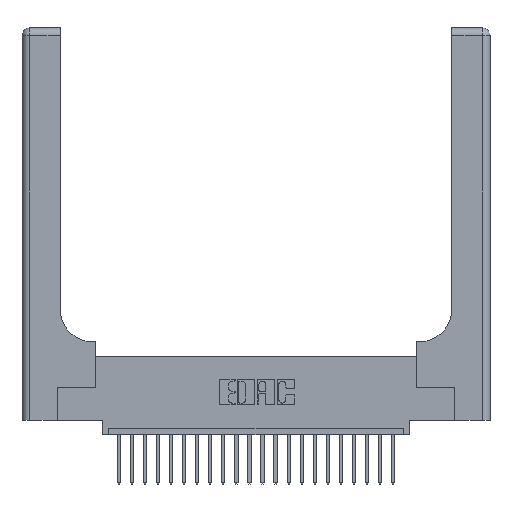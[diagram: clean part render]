
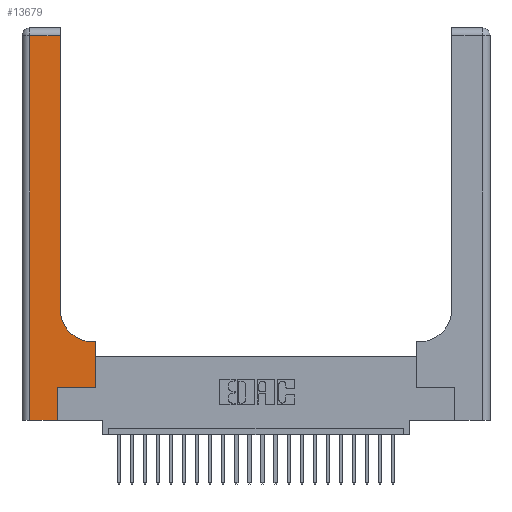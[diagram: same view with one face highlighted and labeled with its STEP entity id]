
A CAD part, top view. The second image highlights one B-rep face of the part: STEP entity #13679.
In plain terms, the highlighted planar face has unit normal (0, 0, 1).
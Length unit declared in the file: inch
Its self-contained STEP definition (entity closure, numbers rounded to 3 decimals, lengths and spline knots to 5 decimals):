
#112 = LINE ( 'NONE', #12360, #22090 ) ;
#316 = CARTESIAN_POINT ( 'NONE',  ( 0.2915, 0.6, 0.37 ) ) ;
#974 = DIRECTION ( 'NONE',  ( 0., -1., 0. ) ) ;
#1729 = EDGE_CURVE ( 'NONE', #9523, #21025, #12473, .T. ) ;
#2277 = CARTESIAN_POINT ( 'NONE',  ( 0.2915, 0.85, 0.37 ) ) ;
#2795 = DIRECTION ( 'NONE',  ( 0., 0., -1. ) ) ;
#3183 = VERTEX_POINT ( 'NONE', #12607 ) ;
#3582 = EDGE_CURVE ( 'NONE', #12081, #3183, #18988, .T. ) ;
#4134 = VERTEX_POINT ( 'NONE', #23323 ) ;
#4288 = VECTOR ( 'NONE', #13110, 39.37008 ) ;
#4659 = EDGE_LOOP ( 'NONE', ( #16622, #6592, #22096, #7080, #19962, #23764, #7042, #21078, #12914 ) ) ;
#5710 = DIRECTION ( 'NONE',  ( 0., 1., 0. ) ) ;
#5900 = AXIS2_PLACEMENT_3D ( 'NONE', #19976, #2795, #10664 ) ;
#6102 = EDGE_CURVE ( 'NONE', #3183, #21782, #10334, .T. ) ;
#6153 = VECTOR ( 'NONE', #13230, 39.37008 ) ;
#6592 = ORIENTED_EDGE ( 'NONE', *, *, #18947, .T. ) ;
#6734 = EDGE_CURVE ( 'NONE', #21782, #21423, #7620, .T. ) ;
#7042 = ORIENTED_EDGE ( 'NONE', *, *, #6734, .T. ) ;
#7080 = ORIENTED_EDGE ( 'NONE', *, *, #23295, .T. ) ;
#7178 = DIRECTION ( 'NONE',  ( 1., 0., 0. ) ) ;
#7620 = LINE ( 'NONE', #17239, #6153 ) ;
#7643 = DIRECTION ( 'NONE',  ( -1., 0., 0. ) ) ;
#8155 = EDGE_CURVE ( 'NONE', #19479, #10838, #112, .T. ) ;
#8750 = CARTESIAN_POINT ( 'NONE',  ( 0.2915, 2.94, 0.37 ) ) ;
#9523 = VERTEX_POINT ( 'NONE', #2277 ) ;
#10334 = LINE ( 'NONE', #15279, #15706 ) ;
#10664 = DIRECTION ( 'NONE',  ( -1., 0., 0. ) ) ;
#10838 = VERTEX_POINT ( 'NONE', #13385 ) ;
#10939 = CARTESIAN_POINT ( 'NONE',  ( 0., 0., 0.37 ) ) ;
#12081 = VERTEX_POINT ( 'NONE', #16821 ) ;
#12098 = DIRECTION ( 'NONE',  ( -1., 0., 0. ) ) ;
#12360 = CARTESIAN_POINT ( 'NONE',  ( 0.06, 3., 0.37 ) ) ;
#12417 = PLANE ( 'NONE',  #5900 ) ;
#12473 = LINE ( 'NONE', #17349, #22562 ) ;
#12574 = LINE ( 'NONE', #316, #21775 ) ;
#12607 = CARTESIAN_POINT ( 'NONE',  ( 0.269, 0.25, 0.37 ) ) ;
#12914 = ORIENTED_EDGE ( 'NONE', *, *, #14063, .T. ) ;
#12995 = DIRECTION ( 'NONE',  ( 0., 0., -1. ) ) ;
#13110 = DIRECTION ( 'NONE',  ( 1., 0., 0. ) ) ;
#13230 = DIRECTION ( 'NONE',  ( 0., 1., 0. ) ) ;
#13385 = CARTESIAN_POINT ( 'NONE',  ( 0.06, 0., 0.37 ) ) ;
#13679 = ADVANCED_FACE ( 'NONE', ( #20587 ), #12417, .F. ) ;
#14063 = EDGE_CURVE ( 'NONE', #4134, #9523, #15872, .T. ) ;
#15234 = LINE ( 'NONE', #19058, #21139 ) ;
#15279 = CARTESIAN_POINT ( 'NONE',  ( 0.269, 0.25, 0.37 ) ) ;
#15706 = VECTOR ( 'NONE', #17365, 39.37008 ) ;
#15872 = CIRCLE ( 'NONE', #20373, 0.25 ) ;
#16622 = ORIENTED_EDGE ( 'NONE', *, *, #1729, .T. ) ;
#16821 = CARTESIAN_POINT ( 'NONE',  ( 0.269, 0., 0.37 ) ) ;
#17072 = CARTESIAN_POINT ( 'NONE',  ( 0.5585, 0.25, 0.37 ) ) ;
#17239 = CARTESIAN_POINT ( 'NONE',  ( 0.5585, 0.25, 0.37 ) ) ;
#17349 = CARTESIAN_POINT ( 'NONE',  ( 0.2915, 3., 0.37 ) ) ;
#17365 = DIRECTION ( 'NONE',  ( 1., 0., 0. ) ) ;
#18696 = CARTESIAN_POINT ( 'NONE',  ( 0.06, 2.94, 0.37 ) ) ;
#18947 = EDGE_CURVE ( 'NONE', #21025, #19479, #15234, .T. ) ;
#18988 = LINE ( 'NONE', #22108, #19579 ) ;
#19058 = CARTESIAN_POINT ( 'NONE',  ( 0., 2.94, 0.37 ) ) ;
#19479 = VERTEX_POINT ( 'NONE', #18696 ) ;
#19579 = VECTOR ( 'NONE', #24164, 39.37008 ) ;
#19817 = CARTESIAN_POINT ( 'NONE',  ( 0.5585, 0.6, 0.37 ) ) ;
#19962 = ORIENTED_EDGE ( 'NONE', *, *, #3582, .T. ) ;
#19976 = CARTESIAN_POINT ( 'NONE',  ( 0., 3., 0.37 ) ) ;
#20373 = AXIS2_PLACEMENT_3D ( 'NONE', #23996, #12995, #7178 ) ;
#20587 = FACE_OUTER_BOUND ( 'NONE', #4659, .T. ) ;
#21025 = VERTEX_POINT ( 'NONE', #8750 ) ;
#21078 = ORIENTED_EDGE ( 'NONE', *, *, #23519, .T. ) ;
#21139 = VECTOR ( 'NONE', #7643, 39.37008 ) ;
#21423 = VERTEX_POINT ( 'NONE', #19817 ) ;
#21479 = LINE ( 'NONE', #10939, #4288 ) ;
#21775 = VECTOR ( 'NONE', #12098, 39.37008 ) ;
#21782 = VERTEX_POINT ( 'NONE', #17072 ) ;
#22090 = VECTOR ( 'NONE', #974, 39.37008 ) ;
#22096 = ORIENTED_EDGE ( 'NONE', *, *, #8155, .T. ) ;
#22108 = CARTESIAN_POINT ( 'NONE',  ( 0.269, 0., 0.37 ) ) ;
#22562 = VECTOR ( 'NONE', #5710, 39.37008 ) ;
#23295 = EDGE_CURVE ( 'NONE', #10838, #12081, #21479, .T. ) ;
#23323 = CARTESIAN_POINT ( 'NONE',  ( 0.5415, 0.6, 0.37 ) ) ;
#23519 = EDGE_CURVE ( 'NONE', #21423, #4134, #12574, .T. ) ;
#23764 = ORIENTED_EDGE ( 'NONE', *, *, #6102, .T. ) ;
#23996 = CARTESIAN_POINT ( 'NONE',  ( 0.5415, 0.85, 0.37 ) ) ;
#24164 = DIRECTION ( 'NONE',  ( 0., 1., 0. ) ) ;
